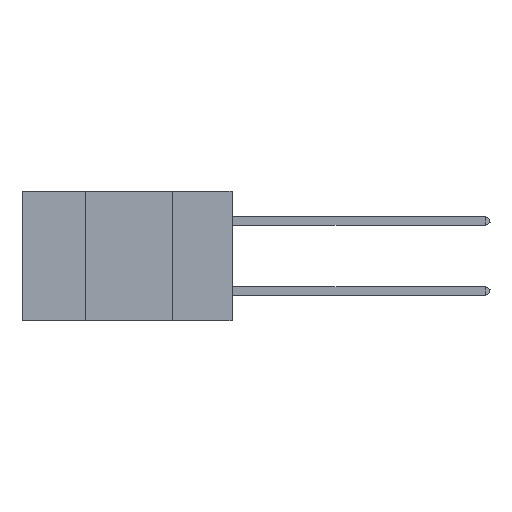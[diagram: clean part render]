
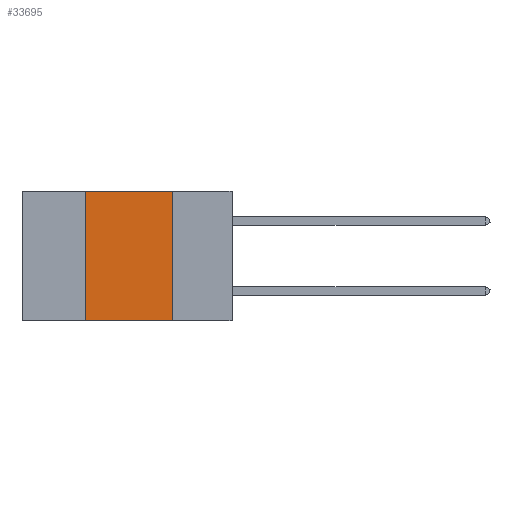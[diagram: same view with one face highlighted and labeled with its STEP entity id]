
A CAD part, left-side view. The second image highlights one B-rep face of the part: STEP entity #33695.
In plain terms, the highlighted planar face has unit normal (-1, 0, 0).
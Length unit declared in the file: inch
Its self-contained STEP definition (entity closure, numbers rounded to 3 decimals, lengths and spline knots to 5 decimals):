
#2010 = LINE ( 'NONE', #7650, #9465 ) ;
#3896 = AXIS2_PLACEMENT_3D ( 'NONE', #28102, #30851, #14599 ) ;
#4366 = ORIENTED_EDGE ( 'NONE', *, *, #31555, .F. ) ;
#5623 = VERTEX_POINT ( 'NONE', #8954 ) ;
#6873 = VERTEX_POINT ( 'NONE', #6916 ) ;
#6916 = CARTESIAN_POINT ( 'NONE',  ( 0., 0.17, -0.37 ) ) ;
#7224 = LINE ( 'NONE', #10923, #8110 ) ;
#7650 = CARTESIAN_POINT ( 'NONE',  ( 0., 0.6, -0.37 ) ) ;
#8110 = VECTOR ( 'NONE', #8178, 39.37008 ) ;
#8178 = DIRECTION ( 'NONE',  ( 0., -1., 0. ) ) ;
#8954 = CARTESIAN_POINT ( 'NONE',  ( 0., 0.42, 0. ) ) ;
#9137 = PLANE ( 'NONE',  #3896 ) ;
#9465 = VECTOR ( 'NONE', #21192, 39.37008 ) ;
#10923 = CARTESIAN_POINT ( 'NONE',  ( 0., 0.6, 0. ) ) ;
#13463 = VECTOR ( 'NONE', #17756, 39.37008 ) ;
#14058 = LINE ( 'NONE', #30615, #20393 ) ;
#14522 = EDGE_CURVE ( 'NONE', #17266, #6873, #2010, .T. ) ;
#14591 = CARTESIAN_POINT ( 'NONE',  ( 0., 0.17, 0. ) ) ;
#14599 = DIRECTION ( 'NONE',  ( 0., 0., -1. ) ) ;
#15055 = CARTESIAN_POINT ( 'NONE',  ( 0., 0.42, 0. ) ) ;
#15598 = CARTESIAN_POINT ( 'NONE',  ( 0., 0.42, -0.37 ) ) ;
#17266 = VERTEX_POINT ( 'NONE', #15598 ) ;
#17756 = DIRECTION ( 'NONE',  ( 0., 0., 1. ) ) ;
#18299 = EDGE_LOOP ( 'NONE', ( #32046, #4366, #22303, #29944 ) ) ;
#18375 = FACE_OUTER_BOUND ( 'NONE', #18299, .T. ) ;
#20393 = VECTOR ( 'NONE', #33435, 39.37008 ) ;
#21192 = DIRECTION ( 'NONE',  ( 0., -1., 0. ) ) ;
#22303 = ORIENTED_EDGE ( 'NONE', *, *, #23610, .F. ) ;
#23610 = EDGE_CURVE ( 'NONE', #17266, #5623, #34215, .T. ) ;
#28102 = CARTESIAN_POINT ( 'NONE',  ( 0., 0.6, 0. ) ) ;
#29944 = ORIENTED_EDGE ( 'NONE', *, *, #14522, .T. ) ;
#30615 = CARTESIAN_POINT ( 'NONE',  ( 0., 0.17, 0. ) ) ;
#30851 = DIRECTION ( 'NONE',  ( 1., 0., 0. ) ) ;
#31555 = EDGE_CURVE ( 'NONE', #5623, #31824, #7224, .T. ) ;
#31778 = EDGE_CURVE ( 'NONE', #31824, #6873, #14058, .T. ) ;
#31824 = VERTEX_POINT ( 'NONE', #14591 ) ;
#32046 = ORIENTED_EDGE ( 'NONE', *, *, #31778, .F. ) ;
#33435 = DIRECTION ( 'NONE',  ( 0., 0., -1. ) ) ;
#33695 = ADVANCED_FACE ( 'NONE', ( #18375 ), #9137, .F. ) ;
#34215 = LINE ( 'NONE', #15055, #13463 ) ;
